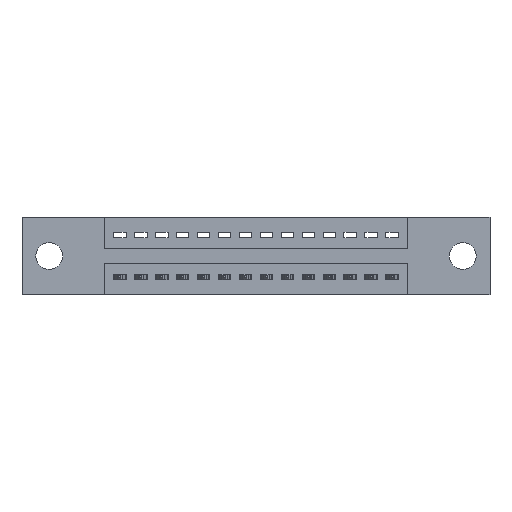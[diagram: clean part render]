
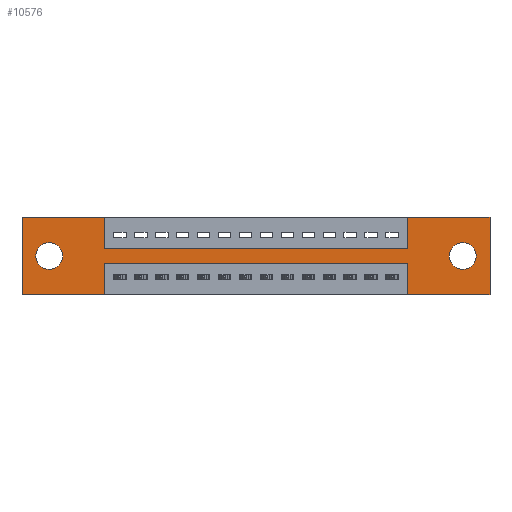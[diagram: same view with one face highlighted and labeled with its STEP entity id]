
A CAD part, front view. The second image highlights one B-rep face of the part: STEP entity #10576.
In plain terms, the highlighted planar face has unit normal (0, -1, 0).
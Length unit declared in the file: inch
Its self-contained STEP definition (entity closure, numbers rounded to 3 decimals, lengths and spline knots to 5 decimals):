
#261 = ORIENTED_EDGE ( 'NONE', *, *, #10227, .T. ) ;
#273 = CARTESIAN_POINT ( 'NONE',  ( 0.13, 0., -0.185 ) ) ;
#405 = VECTOR ( 'NONE', #9969, 39.37008 ) ;
#509 = DIRECTION ( 'NONE',  ( 0., 0., -1. ) ) ;
#614 = LINE ( 'NONE', #6271, #13003 ) ;
#634 = ORIENTED_EDGE ( 'NONE', *, *, #2852, .T. ) ;
#721 = EDGE_LOOP ( 'NONE', ( #8590, #11315, #14057, #9958, #11091, #9671, #4468, #12703, #6492, #3984, #11131, #13214 ) ) ;
#874 = EDGE_LOOP ( 'NONE', ( #5216, #261 ) ) ;
#877 = ORIENTED_EDGE ( 'NONE', *, *, #13084, .T. ) ;
#974 = CARTESIAN_POINT ( 'NONE',  ( 0.3925, 0., -0.22 ) ) ;
#1226 = DIRECTION ( 'NONE',  ( 0., 1., 0. ) ) ;
#1312 = EDGE_CURVE ( 'NONE', #10253, #11510, #8530, .T. ) ;
#1436 = DIRECTION ( 'NONE',  ( -1., 0., 0. ) ) ;
#1444 = CIRCLE ( 'NONE', #5032, 0.064 ) ;
#1589 = CARTESIAN_POINT ( 'NONE',  ( 0.13, 0., -0.121 ) ) ;
#1640 = DIRECTION ( 'NONE',  ( 0., 1., 0. ) ) ;
#1781 = CARTESIAN_POINT ( 'NONE',  ( 2.235, 0., 0. ) ) ;
#1795 = VERTEX_POINT ( 'NONE', #10356 ) ;
#1980 = DIRECTION ( 'NONE',  ( 0., 1., 0. ) ) ;
#2194 = VECTOR ( 'NONE', #1436, 39.37008 ) ;
#2231 = EDGE_CURVE ( 'NONE', #14276, #4127, #8515, .T. ) ;
#2556 = CARTESIAN_POINT ( 'NONE',  ( 0.3925, 0., -0.37 ) ) ;
#2698 = DIRECTION ( 'NONE',  ( 0., 0., 1. ) ) ;
#2715 = VECTOR ( 'NONE', #7164, 39.37008 ) ;
#2743 = CARTESIAN_POINT ( 'NONE',  ( 0., 0., 0. ) ) ;
#2852 = EDGE_CURVE ( 'NONE', #3186, #6046, #1444, .T. ) ;
#3094 = EDGE_CURVE ( 'NONE', #8393, #12606, #614, .T. ) ;
#3186 = VERTEX_POINT ( 'NONE', #9655 ) ;
#3285 = VECTOR ( 'NONE', #10500, 39.37008 ) ;
#3339 = CARTESIAN_POINT ( 'NONE',  ( 0.13, 0., -0.249 ) ) ;
#3399 = LINE ( 'NONE', #11403, #2715 ) ;
#3401 = FACE_OUTER_BOUND ( 'NONE', #721, .T. ) ;
#3478 = LINE ( 'NONE', #8883, #11752 ) ;
#3586 = CARTESIAN_POINT ( 'NONE',  ( 1.8425, 0., -0.37 ) ) ;
#3729 = PLANE ( 'NONE',  #13346 ) ;
#3808 = LINE ( 'NONE', #7224, #10312 ) ;
#3832 = DIRECTION ( 'NONE',  ( 0., 0., 1. ) ) ;
#3868 = VECTOR ( 'NONE', #6794, 39.37008 ) ;
#3974 = VERTEX_POINT ( 'NONE', #13456 ) ;
#3984 = ORIENTED_EDGE ( 'NONE', *, *, #1312, .F. ) ;
#4127 = VERTEX_POINT ( 'NONE', #3586 ) ;
#4190 = VERTEX_POINT ( 'NONE', #6129 ) ;
#4219 = CARTESIAN_POINT ( 'NONE',  ( 0.3925, 0., 0. ) ) ;
#4248 = VERTEX_POINT ( 'NONE', #1589 ) ;
#4274 = CARTESIAN_POINT ( 'NONE',  ( 0., 0., -0.37 ) ) ;
#4341 = AXIS2_PLACEMENT_3D ( 'NONE', #6866, #1640, #3832 ) ;
#4419 = CIRCLE ( 'NONE', #4936, 0.064 ) ;
#4449 = AXIS2_PLACEMENT_3D ( 'NONE', #273, #4709, #5800 ) ;
#4468 = ORIENTED_EDGE ( 'NONE', *, *, #6092, .F. ) ;
#4709 = DIRECTION ( 'NONE',  ( 0., 1., 0. ) ) ;
#4746 = CARTESIAN_POINT ( 'NONE',  ( 0.3925, 0., -0.15 ) ) ;
#4748 = FACE_BOUND ( 'NONE', #12937, .T. ) ;
#4936 = AXIS2_PLACEMENT_3D ( 'NONE', #12884, #1980, #10654 ) ;
#5032 = AXIS2_PLACEMENT_3D ( 'NONE', #13361, #1226, #12064 ) ;
#5087 = DIRECTION ( 'NONE',  ( 0., 0., -1. ) ) ;
#5167 = LINE ( 'NONE', #13902, #3285 ) ;
#5194 = LINE ( 'NONE', #2743, #5514 ) ;
#5198 = VERTEX_POINT ( 'NONE', #3339 ) ;
#5204 = LINE ( 'NONE', #5315, #6045 ) ;
#5216 = ORIENTED_EDGE ( 'NONE', *, *, #10765, .T. ) ;
#5234 = VECTOR ( 'NONE', #14208, 39.37008 ) ;
#5315 = CARTESIAN_POINT ( 'NONE',  ( 0., 0., 0. ) ) ;
#5413 = VERTEX_POINT ( 'NONE', #4746 ) ;
#5514 = VECTOR ( 'NONE', #2698, 39.37008 ) ;
#5792 = CARTESIAN_POINT ( 'NONE',  ( 2.235, 0., 0. ) ) ;
#5800 = DIRECTION ( 'NONE',  ( 0., 0., 1. ) ) ;
#6045 = VECTOR ( 'NONE', #9762, 39.37008 ) ;
#6046 = VERTEX_POINT ( 'NONE', #6224 ) ;
#6092 = EDGE_CURVE ( 'NONE', #3974, #4190, #5167, .T. ) ;
#6129 = CARTESIAN_POINT ( 'NONE',  ( 1.8425, 0., 0. ) ) ;
#6224 = CARTESIAN_POINT ( 'NONE',  ( 2.105, 0., -0.249 ) ) ;
#6271 = CARTESIAN_POINT ( 'NONE',  ( 0.3925, 0., -0.37 ) ) ;
#6361 = EDGE_CURVE ( 'NONE', #5413, #3974, #3399, .T. ) ;
#6492 = ORIENTED_EDGE ( 'NONE', *, *, #13864, .F. ) ;
#6657 = CARTESIAN_POINT ( 'NONE',  ( 1.8425, 0., -0.37 ) ) ;
#6676 = EDGE_CURVE ( 'NONE', #1795, #8393, #10031, .T. ) ;
#6794 = DIRECTION ( 'NONE',  ( 0., 0., -1. ) ) ;
#6866 = CARTESIAN_POINT ( 'NONE',  ( 0.13, 0., -0.185 ) ) ;
#6945 = EDGE_CURVE ( 'NONE', #7463, #14276, #7776, .T. ) ;
#7018 = DIRECTION ( 'NONE',  ( 0., 0., -1. ) ) ;
#7164 = DIRECTION ( 'NONE',  ( 1., 0., 0. ) ) ;
#7224 = CARTESIAN_POINT ( 'NONE',  ( 0.3925, 0., 0. ) ) ;
#7463 = VERTEX_POINT ( 'NONE', #1781 ) ;
#7570 = VERTEX_POINT ( 'NONE', #4274 ) ;
#7776 = LINE ( 'NONE', #5792, #3868 ) ;
#8393 = VERTEX_POINT ( 'NONE', #11302 ) ;
#8515 = LINE ( 'NONE', #13674, #2194 ) ;
#8530 = LINE ( 'NONE', #8592, #9402 ) ;
#8590 = ORIENTED_EDGE ( 'NONE', *, *, #3094, .F. ) ;
#8592 = CARTESIAN_POINT ( 'NONE',  ( 0., 0., 0. ) ) ;
#8695 = FACE_BOUND ( 'NONE', #874, .T. ) ;
#8883 = CARTESIAN_POINT ( 'NONE',  ( 0., 0., -0.37 ) ) ;
#9241 = CARTESIAN_POINT ( 'NONE',  ( 0., 0., 0. ) ) ;
#9259 = CIRCLE ( 'NONE', #4341, 0.064 ) ;
#9402 = VECTOR ( 'NONE', #10682, 39.37008 ) ;
#9655 = CARTESIAN_POINT ( 'NONE',  ( 2.105, 0., -0.121 ) ) ;
#9671 = ORIENTED_EDGE ( 'NONE', *, *, #13622, .F. ) ;
#9762 = DIRECTION ( 'NONE',  ( 1., 0., 0. ) ) ;
#9958 = ORIENTED_EDGE ( 'NONE', *, *, #2231, .F. ) ;
#9969 = DIRECTION ( 'NONE',  ( 0., 0., 1. ) ) ;
#10031 = LINE ( 'NONE', #974, #5234 ) ;
#10227 = EDGE_CURVE ( 'NONE', #5198, #4248, #9259, .T. ) ;
#10253 = VERTEX_POINT ( 'NONE', #9241 ) ;
#10312 = VECTOR ( 'NONE', #509, 39.37008 ) ;
#10356 = CARTESIAN_POINT ( 'NONE',  ( 1.8425, 0., -0.22 ) ) ;
#10500 = DIRECTION ( 'NONE',  ( 0., 0., 1. ) ) ;
#10576 = ADVANCED_FACE ( 'NONE', ( #4748, #8695, #3401 ), #3729, .T. ) ;
#10654 = DIRECTION ( 'NONE',  ( 0., 0., -1. ) ) ;
#10682 = DIRECTION ( 'NONE',  ( 1., 0., 0. ) ) ;
#10765 = EDGE_CURVE ( 'NONE', #4248, #5198, #11117, .T. ) ;
#11091 = ORIENTED_EDGE ( 'NONE', *, *, #6945, .F. ) ;
#11117 = CIRCLE ( 'NONE', #4449, 0.064 ) ;
#11131 = ORIENTED_EDGE ( 'NONE', *, *, #12515, .F. ) ;
#11181 = CARTESIAN_POINT ( 'NONE',  ( 2.235, 0., -0.37 ) ) ;
#11227 = CARTESIAN_POINT ( 'NONE',  ( 0., 0., -0.37 ) ) ;
#11302 = CARTESIAN_POINT ( 'NONE',  ( 0.3925, 0., -0.22 ) ) ;
#11315 = ORIENTED_EDGE ( 'NONE', *, *, #6676, .F. ) ;
#11403 = CARTESIAN_POINT ( 'NONE',  ( 0.3925, 0., -0.15 ) ) ;
#11432 = EDGE_CURVE ( 'NONE', #4127, #1795, #14069, .T. ) ;
#11510 = VERTEX_POINT ( 'NONE', #4219 ) ;
#11752 = VECTOR ( 'NONE', #13669, 39.37008 ) ;
#12064 = DIRECTION ( 'NONE',  ( 0., 0., -1. ) ) ;
#12289 = EDGE_CURVE ( 'NONE', #12606, #7570, #3478, .T. ) ;
#12408 = DIRECTION ( 'NONE',  ( 0., -1., 0. ) ) ;
#12515 = EDGE_CURVE ( 'NONE', #7570, #10253, #5194, .T. ) ;
#12606 = VERTEX_POINT ( 'NONE', #2556 ) ;
#12703 = ORIENTED_EDGE ( 'NONE', *, *, #6361, .F. ) ;
#12884 = CARTESIAN_POINT ( 'NONE',  ( 2.105, 0., -0.185 ) ) ;
#12937 = EDGE_LOOP ( 'NONE', ( #634, #877 ) ) ;
#13003 = VECTOR ( 'NONE', #5087, 39.37008 ) ;
#13084 = EDGE_CURVE ( 'NONE', #6046, #3186, #4419, .T. ) ;
#13214 = ORIENTED_EDGE ( 'NONE', *, *, #12289, .F. ) ;
#13346 = AXIS2_PLACEMENT_3D ( 'NONE', #11227, #12408, #7018 ) ;
#13361 = CARTESIAN_POINT ( 'NONE',  ( 2.105, 0., -0.185 ) ) ;
#13456 = CARTESIAN_POINT ( 'NONE',  ( 1.8425, 0., -0.15 ) ) ;
#13622 = EDGE_CURVE ( 'NONE', #4190, #7463, #5204, .T. ) ;
#13669 = DIRECTION ( 'NONE',  ( -1., 0., 0. ) ) ;
#13674 = CARTESIAN_POINT ( 'NONE',  ( 0., 0., -0.37 ) ) ;
#13864 = EDGE_CURVE ( 'NONE', #11510, #5413, #3808, .T. ) ;
#13902 = CARTESIAN_POINT ( 'NONE',  ( 1.8425, 0., 0. ) ) ;
#14057 = ORIENTED_EDGE ( 'NONE', *, *, #11432, .F. ) ;
#14069 = LINE ( 'NONE', #6657, #405 ) ;
#14208 = DIRECTION ( 'NONE',  ( -1., 0., 0. ) ) ;
#14276 = VERTEX_POINT ( 'NONE', #11181 ) ;
